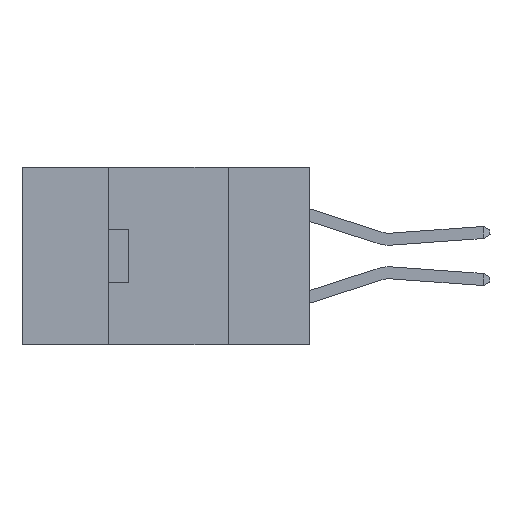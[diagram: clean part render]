
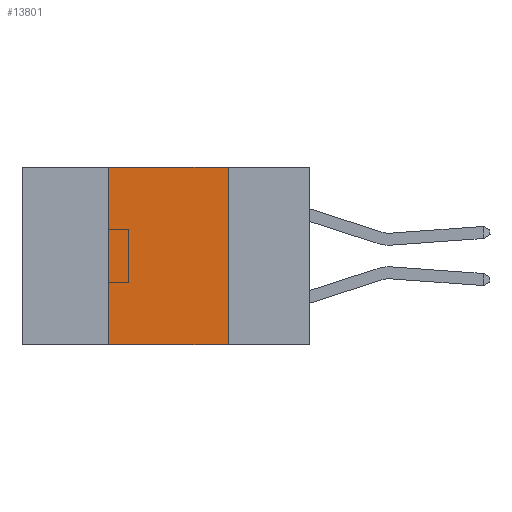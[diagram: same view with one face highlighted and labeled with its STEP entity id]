
A CAD part, left-side view. The second image highlights one B-rep face of the part: STEP entity #13801.
In plain terms, the highlighted planar face has unit normal (-1, 0, 0).
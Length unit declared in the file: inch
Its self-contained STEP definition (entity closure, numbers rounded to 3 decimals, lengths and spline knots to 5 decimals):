
#123 = CARTESIAN_POINT ( 'NONE',  ( 0., 0.6, 0. ) ) ;
#848 = LINE ( 'NONE', #26838, #11853 ) ;
#1259 = CARTESIAN_POINT ( 'NONE',  ( 0., 0.42, -0.37 ) ) ;
#2949 = FACE_OUTER_BOUND ( 'NONE', #20533, .T. ) ;
#3522 = DIRECTION ( 'NONE',  ( 0., 0., 1. ) ) ;
#4243 = ORIENTED_EDGE ( 'NONE', *, *, #17402, .F. ) ;
#4632 = DIRECTION ( 'NONE',  ( 0., 0., -1. ) ) ;
#4918 = ORIENTED_EDGE ( 'NONE', *, *, #20309, .F. ) ;
#7172 = CARTESIAN_POINT ( 'NONE',  ( 0., 0.42, 0. ) ) ;
#7207 = DIRECTION ( 'NONE',  ( 0., -1., 0. ) ) ;
#7549 = VERTEX_POINT ( 'NONE', #12403 ) ;
#9909 = CARTESIAN_POINT ( 'NONE',  ( 0., 0.42, -0.37 ) ) ;
#10131 = LINE ( 'NONE', #21980, #15924 ) ;
#11452 = LINE ( 'NONE', #1259, #28273 ) ;
#11853 = VECTOR ( 'NONE', #7207, 39.37008 ) ;
#12403 = CARTESIAN_POINT ( 'NONE',  ( 0., 0.17, -0.37 ) ) ;
#12484 = DIRECTION ( 'NONE',  ( 0., 0., -1. ) ) ;
#13801 = ADVANCED_FACE ( 'NONE', ( #2949 ), #15497, .F. ) ;
#14386 = EDGE_CURVE ( 'NONE', #17973, #7549, #848, .T. ) ;
#15071 = LINE ( 'NONE', #18996, #25385 ) ;
#15157 = CARTESIAN_POINT ( 'NONE',  ( 0., 0.17, 0. ) ) ;
#15497 = PLANE ( 'NONE',  #19249 ) ;
#15924 = VECTOR ( 'NONE', #21884, 39.37008 ) ;
#17402 = EDGE_CURVE ( 'NONE', #20242, #7549, #15071, .T. ) ;
#17680 = DIRECTION ( 'NONE',  ( 1., 0., 0. ) ) ;
#17884 = ORIENTED_EDGE ( 'NONE', *, *, #22304, .F. ) ;
#17973 = VERTEX_POINT ( 'NONE', #9909 ) ;
#18996 = CARTESIAN_POINT ( 'NONE',  ( 0., 0.17, -0.37 ) ) ;
#19249 = AXIS2_PLACEMENT_3D ( 'NONE', #123, #17680, #4632 ) ;
#20242 = VERTEX_POINT ( 'NONE', #15157 ) ;
#20309 = EDGE_CURVE ( 'NONE', #24814, #20242, #10131, .T. ) ;
#20533 = EDGE_LOOP ( 'NONE', ( #4243, #4918, #17884, #23738 ) ) ;
#21884 = DIRECTION ( 'NONE',  ( 0., -1., 0. ) ) ;
#21980 = CARTESIAN_POINT ( 'NONE',  ( 0., 0.6, 0. ) ) ;
#22304 = EDGE_CURVE ( 'NONE', #17973, #24814, #11452, .T. ) ;
#23738 = ORIENTED_EDGE ( 'NONE', *, *, #14386, .T. ) ;
#24814 = VERTEX_POINT ( 'NONE', #7172 ) ;
#25385 = VECTOR ( 'NONE', #12484, 39.37008 ) ;
#26838 = CARTESIAN_POINT ( 'NONE',  ( 0., 0.6, -0.37 ) ) ;
#28273 = VECTOR ( 'NONE', #3522, 39.37008 ) ;
